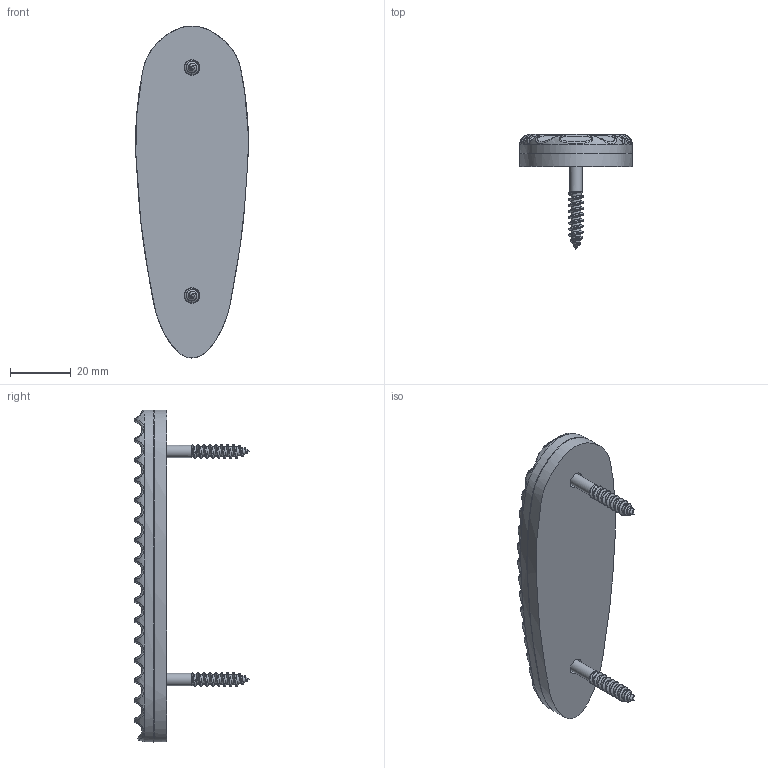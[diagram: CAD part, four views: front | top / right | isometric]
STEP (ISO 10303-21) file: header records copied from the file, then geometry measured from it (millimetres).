
FILE_DESCRIPTION(/* description */ (''),/* implementation_level */ '2;1');
FILE_NAME(/* name */ 'Stock Endplate v4.step',/* time_stamp */ '2020-08-21T23:40:40-04:00',/* author */ (''),/* organization */ (''),/* preprocessor_version */ 'ST-DEVELOPER v18.1',/* originating_system */ 'Autodesk Translation Framework v9.3.0.1241',/* authorisation */ '');
FILE_SCHEMA (('AUTOMOTIVE_DESIGN { 1 0 10303 214 3 1 1 }'));
Length unit declared in the file: millimetre
Products named in the file (3): Stock Endplate; 93360A609; Endplate
Assembly tree (3 placements, depth 2):
  Stock Endplate
    93360A609  x2
    Endplate
Bounding box: 37.27 x 38.08 x 109.75 mm (x, y, z)
Volume: 28632.9 mm3; surface area: 11292.8 mm2
Topology: 3 solids, 3 shells, 236 faces, 567 edges, 339 vertices
Faces by surface type: cylinder 78, plane 65, bspline 53, cone 16, sphere 14, torus 10
Full cylindrical faces by diameter (mm): 3.258 x12, 4.042 x2, 5.2 x2, 9.271 x2, 10.271 x2
Entity records: 15123 total; most frequent: CARTESIAN_POINT 11123, ORIENTED_EDGE 874, DIRECTION 730, EDGE_CURVE 437, AXIS2_PLACEMENT_3D 298, VERTEX_POINT 256, EDGE_LOOP 193, FACE_OUTER_BOUND 187
